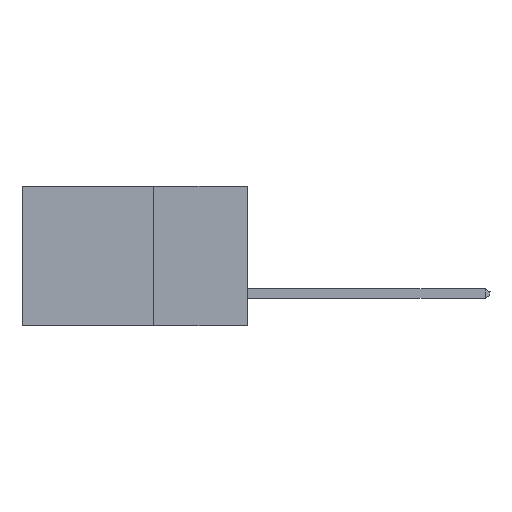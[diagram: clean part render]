
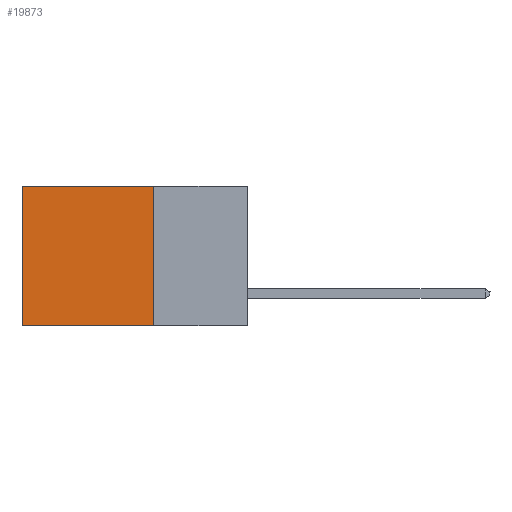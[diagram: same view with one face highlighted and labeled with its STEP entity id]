
A CAD part, left-side view. The second image highlights one B-rep face of the part: STEP entity #19873.
In plain terms, the highlighted planar face has unit normal (-1, 0, 0).
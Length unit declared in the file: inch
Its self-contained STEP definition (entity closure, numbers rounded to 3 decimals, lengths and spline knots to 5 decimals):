
#1217 = DIRECTION ( 'NONE',  ( 0., 0., -1. ) ) ;
#1450 = ORIENTED_EDGE ( 'NONE', *, *, #10196, .F. ) ;
#2190 = ORIENTED_EDGE ( 'NONE', *, *, #19313, .T. ) ;
#2816 = CARTESIAN_POINT ( 'NONE',  ( 0.2615, 0.25, -0.37 ) ) ;
#2842 = VERTEX_POINT ( 'NONE', #15933 ) ;
#2928 = FACE_OUTER_BOUND ( 'NONE', #10528, .T. ) ;
#3043 = PLANE ( 'NONE',  #9637 ) ;
#3416 = LINE ( 'NONE', #10303, #16102 ) ;
#4400 = CARTESIAN_POINT ( 'NONE',  ( 0.2615, 0.6, 0. ) ) ;
#5500 = CARTESIAN_POINT ( 'NONE',  ( 0.2615, 0.6, -0.37 ) ) ;
#8254 = DIRECTION ( 'NONE',  ( 0., 0., -1. ) ) ;
#8340 = DIRECTION ( 'NONE',  ( 1., 0., 0. ) ) ;
#9637 = AXIS2_PLACEMENT_3D ( 'NONE', #2816, #8340, #1217 ) ;
#10196 = EDGE_CURVE ( 'NONE', #2842, #19832, #13339, .T. ) ;
#10303 = CARTESIAN_POINT ( 'NONE',  ( 0.2615, 0.25, -0.37 ) ) ;
#10528 = EDGE_LOOP ( 'NONE', ( #14074, #19294, #1450, #2190 ) ) ;
#10881 = VERTEX_POINT ( 'NONE', #12689 ) ;
#11542 = EDGE_CURVE ( 'NONE', #19832, #10881, #3416, .T. ) ;
#11666 = EDGE_CURVE ( 'NONE', #12688, #10881, #20980, .T. ) ;
#12294 = DIRECTION ( 'NONE',  ( 0., 1., 0. ) ) ;
#12385 = DIRECTION ( 'NONE',  ( 0., 0., -1. ) ) ;
#12688 = VERTEX_POINT ( 'NONE', #4400 ) ;
#12689 = CARTESIAN_POINT ( 'NONE',  ( 0.2615, 0.6, -0.37 ) ) ;
#13339 = LINE ( 'NONE', #15787, #21603 ) ;
#14074 = ORIENTED_EDGE ( 'NONE', *, *, #11666, .T. ) ;
#15249 = CARTESIAN_POINT ( 'NONE',  ( 0.2615, 0.25, 0. ) ) ;
#15393 = VECTOR ( 'NONE', #12294, 39.37008 ) ;
#15787 = CARTESIAN_POINT ( 'NONE',  ( 0.2615, 0.25, -0.37 ) ) ;
#15933 = CARTESIAN_POINT ( 'NONE',  ( 0.2615, 0.25, 0. ) ) ;
#15967 = CARTESIAN_POINT ( 'NONE',  ( 0.2615, 0.25, -0.37 ) ) ;
#16102 = VECTOR ( 'NONE', #17183, 39.37008 ) ;
#16945 = LINE ( 'NONE', #15249, #15393 ) ;
#17183 = DIRECTION ( 'NONE',  ( 0., 1., 0. ) ) ;
#19294 = ORIENTED_EDGE ( 'NONE', *, *, #11542, .F. ) ;
#19313 = EDGE_CURVE ( 'NONE', #2842, #12688, #16945, .T. ) ;
#19832 = VERTEX_POINT ( 'NONE', #15967 ) ;
#19873 = ADVANCED_FACE ( 'NONE', ( #2928 ), #3043, .F. ) ;
#20980 = LINE ( 'NONE', #5500, #22304 ) ;
#21603 = VECTOR ( 'NONE', #8254, 39.37008 ) ;
#22304 = VECTOR ( 'NONE', #12385, 39.37008 ) ;
